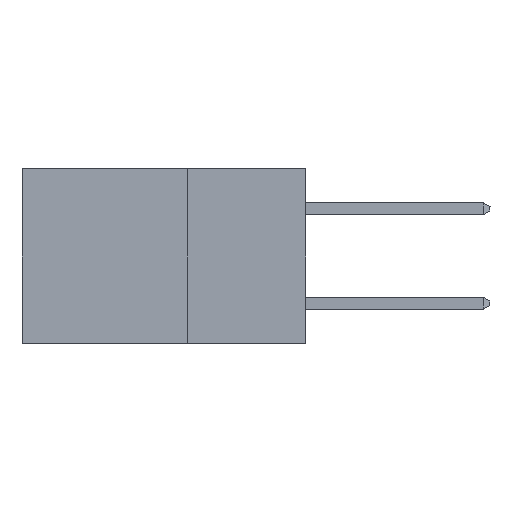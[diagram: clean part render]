
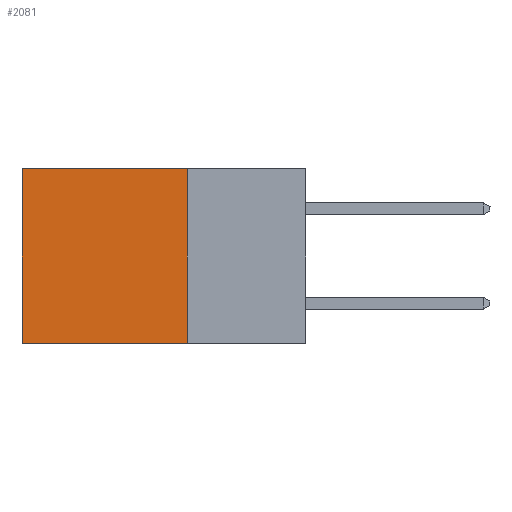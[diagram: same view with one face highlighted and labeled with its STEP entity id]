
A CAD part, left-side view. The second image highlights one B-rep face of the part: STEP entity #2081.
In plain terms, the highlighted planar face has unit normal (-1, 0, 0).
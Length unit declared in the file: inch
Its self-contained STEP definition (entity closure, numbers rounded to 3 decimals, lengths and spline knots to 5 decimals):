
#1040 = EDGE_LOOP ( 'NONE', ( #16222, #14551, #13927, #9261 ) ) ;
#2081 = ADVANCED_FACE ( 'NONE', ( #16026 ), #18552, .F. ) ;
#2293 = CARTESIAN_POINT ( 'NONE',  ( 0.2615, 0.6, -0.37 ) ) ;
#2352 = DIRECTION ( 'NONE',  ( 0., 0., -1. ) ) ;
#2502 = LINE ( 'NONE', #4131, #7375 ) ;
#3908 = EDGE_CURVE ( 'NONE', #4084, #8362, #2502, .T. ) ;
#3928 = AXIS2_PLACEMENT_3D ( 'NONE', #23481, #23098, #22786 ) ;
#3950 = EDGE_CURVE ( 'NONE', #8362, #17002, #12175, .T. ) ;
#4084 = VERTEX_POINT ( 'NONE', #24866 ) ;
#4131 = CARTESIAN_POINT ( 'NONE',  ( 0.2615, 0.25, 0. ) ) ;
#4391 = DIRECTION ( 'NONE',  ( 0., 1., 0. ) ) ;
#5339 = EDGE_CURVE ( 'NONE', #7086, #17002, #5653, .T. ) ;
#5653 = LINE ( 'NONE', #16452, #26089 ) ;
#6445 = CARTESIAN_POINT ( 'NONE',  ( 0.2615, 0.6, 0. ) ) ;
#7086 = VERTEX_POINT ( 'NONE', #17812 ) ;
#7375 = VECTOR ( 'NONE', #4391, 39.37008 ) ;
#8362 = VERTEX_POINT ( 'NONE', #6445 ) ;
#9261 = ORIENTED_EDGE ( 'NONE', *, *, #3908, .T. ) ;
#9608 = DIRECTION ( 'NONE',  ( 0., 0., -1. ) ) ;
#11535 = VECTOR ( 'NONE', #2352, 39.37008 ) ;
#12175 = LINE ( 'NONE', #2293, #11535 ) ;
#13738 = CARTESIAN_POINT ( 'NONE',  ( 0.2615, 0.25, -0.37 ) ) ;
#13927 = ORIENTED_EDGE ( 'NONE', *, *, #20132, .F. ) ;
#14014 = VECTOR ( 'NONE', #9608, 39.37008 ) ;
#14551 = ORIENTED_EDGE ( 'NONE', *, *, #5339, .F. ) ;
#16026 = FACE_OUTER_BOUND ( 'NONE', #1040, .T. ) ;
#16222 = ORIENTED_EDGE ( 'NONE', *, *, #3950, .T. ) ;
#16452 = CARTESIAN_POINT ( 'NONE',  ( 0.2615, 0.25, -0.37 ) ) ;
#17002 = VERTEX_POINT ( 'NONE', #17491 ) ;
#17491 = CARTESIAN_POINT ( 'NONE',  ( 0.2615, 0.6, -0.37 ) ) ;
#17812 = CARTESIAN_POINT ( 'NONE',  ( 0.2615, 0.25, -0.37 ) ) ;
#18504 = DIRECTION ( 'NONE',  ( 0., 1., 0. ) ) ;
#18552 = PLANE ( 'NONE',  #3928 ) ;
#19465 = LINE ( 'NONE', #13738, #14014 ) ;
#20132 = EDGE_CURVE ( 'NONE', #4084, #7086, #19465, .T. ) ;
#22786 = DIRECTION ( 'NONE',  ( 0., 0., -1. ) ) ;
#23098 = DIRECTION ( 'NONE',  ( 1., 0., 0. ) ) ;
#23481 = CARTESIAN_POINT ( 'NONE',  ( 0.2615, 0.25, -0.37 ) ) ;
#24866 = CARTESIAN_POINT ( 'NONE',  ( 0.2615, 0.25, 0. ) ) ;
#26089 = VECTOR ( 'NONE', #18504, 39.37008 ) ;
